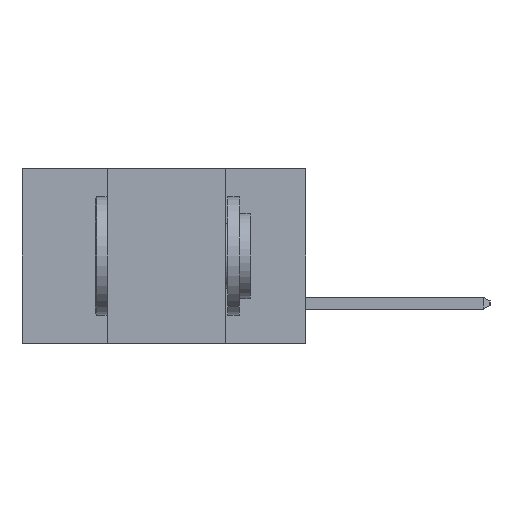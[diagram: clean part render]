
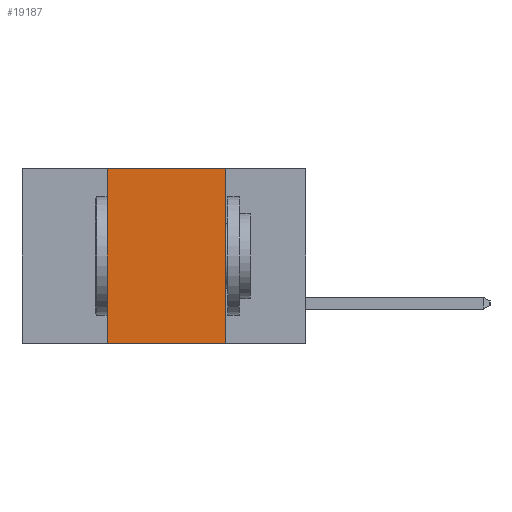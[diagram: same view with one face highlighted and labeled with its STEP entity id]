
A CAD part, left-side view. The second image highlights one B-rep face of the part: STEP entity #19187.
In plain terms, the highlighted planar face has unit normal (-1, 0, 0).
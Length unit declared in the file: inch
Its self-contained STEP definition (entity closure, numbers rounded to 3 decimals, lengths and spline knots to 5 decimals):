
#915 = EDGE_LOOP ( 'NONE', ( #8653, #17865, #6640, #10800 ) ) ;
#1221 = DIRECTION ( 'NONE',  ( 0., 0., -1. ) ) ;
#1922 = EDGE_CURVE ( 'NONE', #4108, #19591, #19302, .T. ) ;
#2151 = VECTOR ( 'NONE', #10917, 39.37008 ) ;
#2634 = LINE ( 'NONE', #11018, #2151 ) ;
#2730 = CARTESIAN_POINT ( 'NONE',  ( 0., 0.6, 0. ) ) ;
#3760 = CARTESIAN_POINT ( 'NONE',  ( 0., 0.17, -0.37 ) ) ;
#4041 = EDGE_CURVE ( 'NONE', #4108, #10619, #2634, .T. ) ;
#4108 = VERTEX_POINT ( 'NONE', #8814 ) ;
#4517 = VERTEX_POINT ( 'NONE', #8967 ) ;
#5804 = DIRECTION ( 'NONE',  ( 0., -1., 0. ) ) ;
#5850 = CARTESIAN_POINT ( 'NONE',  ( 0., 0.6, 0. ) ) ;
#5942 = EDGE_CURVE ( 'NONE', #4517, #19591, #12507, .T. ) ;
#6640 = ORIENTED_EDGE ( 'NONE', *, *, #4041, .F. ) ;
#8653 = ORIENTED_EDGE ( 'NONE', *, *, #5942, .F. ) ;
#8692 = CARTESIAN_POINT ( 'NONE',  ( 0., 0.42, 0. ) ) ;
#8814 = CARTESIAN_POINT ( 'NONE',  ( 0., 0.42, -0.37 ) ) ;
#8967 = CARTESIAN_POINT ( 'NONE',  ( 0., 0.17, 0. ) ) ;
#9178 = VECTOR ( 'NONE', #5804, 39.37008 ) ;
#10522 = DIRECTION ( 'NONE',  ( 1., 0., 0. ) ) ;
#10615 = CARTESIAN_POINT ( 'NONE',  ( 0., 0.6, -0.37 ) ) ;
#10619 = VERTEX_POINT ( 'NONE', #8692 ) ;
#10651 = DIRECTION ( 'NONE',  ( 0., -1., 0. ) ) ;
#10783 = AXIS2_PLACEMENT_3D ( 'NONE', #2730, #10522, #1221 ) ;
#10800 = ORIENTED_EDGE ( 'NONE', *, *, #1922, .T. ) ;
#10871 = EDGE_CURVE ( 'NONE', #10619, #4517, #17702, .T. ) ;
#10917 = DIRECTION ( 'NONE',  ( 0., 0., 1. ) ) ;
#11018 = CARTESIAN_POINT ( 'NONE',  ( 0., 0.42, -0.37 ) ) ;
#11403 = VECTOR ( 'NONE', #10651, 39.37008 ) ;
#12507 = LINE ( 'NONE', #16805, #16504 ) ;
#16401 = FACE_OUTER_BOUND ( 'NONE', #915, .T. ) ;
#16504 = VECTOR ( 'NONE', #16604, 39.37008 ) ;
#16604 = DIRECTION ( 'NONE',  ( 0., 0., -1. ) ) ;
#16805 = CARTESIAN_POINT ( 'NONE',  ( 0., 0.17, -0.37 ) ) ;
#17702 = LINE ( 'NONE', #5850, #9178 ) ;
#17865 = ORIENTED_EDGE ( 'NONE', *, *, #10871, .F. ) ;
#19187 = ADVANCED_FACE ( 'NONE', ( #16401 ), #19402, .F. ) ;
#19302 = LINE ( 'NONE', #10615, #11403 ) ;
#19402 = PLANE ( 'NONE',  #10783 ) ;
#19591 = VERTEX_POINT ( 'NONE', #3760 ) ;
